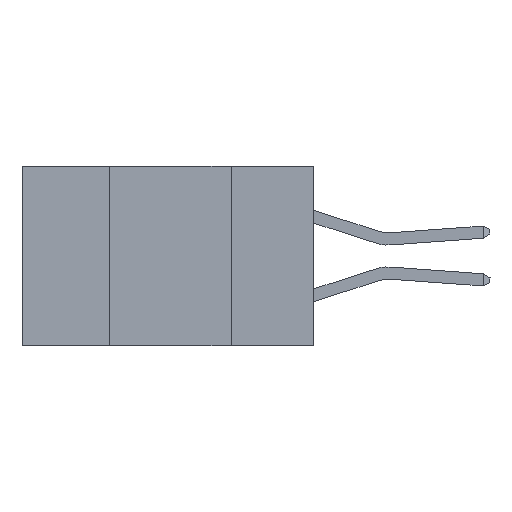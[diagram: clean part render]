
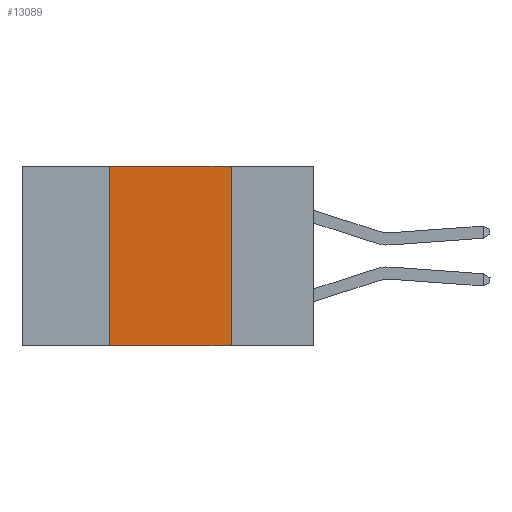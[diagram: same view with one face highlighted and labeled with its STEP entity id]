
A CAD part, left-side view. The second image highlights one B-rep face of the part: STEP entity #13089.
In plain terms, the highlighted planar face has unit normal (-1, 0, 0).
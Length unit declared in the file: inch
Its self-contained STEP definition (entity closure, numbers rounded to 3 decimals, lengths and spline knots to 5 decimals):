
#125 = CARTESIAN_POINT ( 'NONE',  ( 0., 0.6, 0. ) ) ;
#209 = PLANE ( 'NONE',  #23175 ) ;
#326 = VECTOR ( 'NONE', #24019, 39.37008 ) ;
#1790 = CARTESIAN_POINT ( 'NONE',  ( 0., 0.6, 0. ) ) ;
#1873 = EDGE_CURVE ( 'NONE', #19645, #23298, #5564, .T. ) ;
#4032 = ORIENTED_EDGE ( 'NONE', *, *, #24105, .F. ) ;
#4162 = DIRECTION ( 'NONE',  ( 0., 0., -1. ) ) ;
#5259 = ORIENTED_EDGE ( 'NONE', *, *, #10446, .F. ) ;
#5564 = LINE ( 'NONE', #22082, #326 ) ;
#5836 = EDGE_CURVE ( 'NONE', #19645, #13533, #18776, .T. ) ;
#5966 = CARTESIAN_POINT ( 'NONE',  ( 0., 0.17, 0. ) ) ;
#6268 = CARTESIAN_POINT ( 'NONE',  ( 0., 0.42, 0. ) ) ;
#9208 = CARTESIAN_POINT ( 'NONE',  ( 0., 0.17, -0.37 ) ) ;
#9289 = VECTOR ( 'NONE', #17514, 39.37008 ) ;
#10446 = EDGE_CURVE ( 'NONE', #13533, #11316, #15089, .T. ) ;
#11316 = VERTEX_POINT ( 'NONE', #16034 ) ;
#11665 = VECTOR ( 'NONE', #21542, 39.37008 ) ;
#13089 = ADVANCED_FACE ( 'NONE', ( #19400 ), #209, .F. ) ;
#13533 = VERTEX_POINT ( 'NONE', #22990 ) ;
#15089 = LINE ( 'NONE', #1790, #9289 ) ;
#15661 = ORIENTED_EDGE ( 'NONE', *, *, #5836, .F. ) ;
#15867 = DIRECTION ( 'NONE',  ( 1., 0., 0. ) ) ;
#15967 = DIRECTION ( 'NONE',  ( 0., 0., 1. ) ) ;
#16034 = CARTESIAN_POINT ( 'NONE',  ( 0., 0.17, 0. ) ) ;
#16779 = EDGE_LOOP ( 'NONE', ( #4032, #5259, #15661, #23274 ) ) ;
#17466 = LINE ( 'NONE', #5966, #11665 ) ;
#17514 = DIRECTION ( 'NONE',  ( 0., -1., 0. ) ) ;
#18776 = LINE ( 'NONE', #6268, #23933 ) ;
#19400 = FACE_OUTER_BOUND ( 'NONE', #16779, .T. ) ;
#19645 = VERTEX_POINT ( 'NONE', #20469 ) ;
#20469 = CARTESIAN_POINT ( 'NONE',  ( 0., 0.42, -0.37 ) ) ;
#21542 = DIRECTION ( 'NONE',  ( 0., 0., -1. ) ) ;
#22082 = CARTESIAN_POINT ( 'NONE',  ( 0., 0.6, -0.37 ) ) ;
#22990 = CARTESIAN_POINT ( 'NONE',  ( 0., 0.42, 0. ) ) ;
#23175 = AXIS2_PLACEMENT_3D ( 'NONE', #125, #15867, #4162 ) ;
#23274 = ORIENTED_EDGE ( 'NONE', *, *, #1873, .T. ) ;
#23298 = VERTEX_POINT ( 'NONE', #9208 ) ;
#23933 = VECTOR ( 'NONE', #15967, 39.37008 ) ;
#24019 = DIRECTION ( 'NONE',  ( 0., -1., 0. ) ) ;
#24105 = EDGE_CURVE ( 'NONE', #11316, #23298, #17466, .T. ) ;
